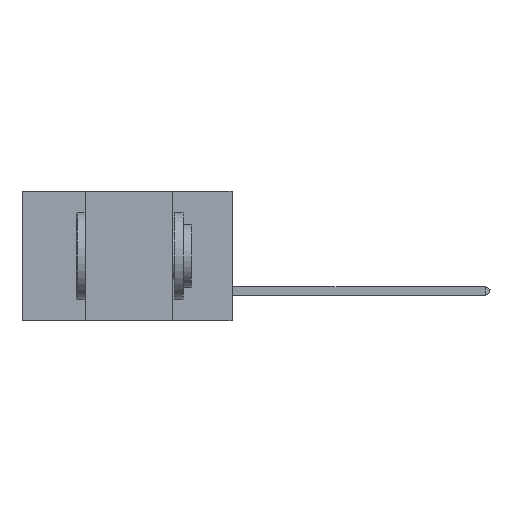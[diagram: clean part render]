
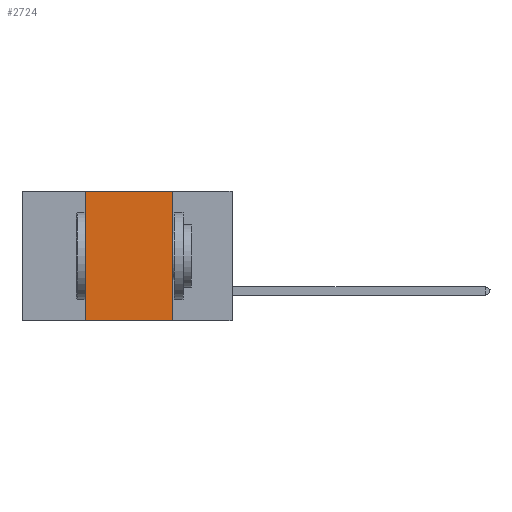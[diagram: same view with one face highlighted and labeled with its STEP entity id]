
A CAD part, left-side view. The second image highlights one B-rep face of the part: STEP entity #2724.
In plain terms, the highlighted planar face has unit normal (-1, 0, 0).
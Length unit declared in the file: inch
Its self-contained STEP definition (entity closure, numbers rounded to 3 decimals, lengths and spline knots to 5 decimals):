
#9 = CARTESIAN_POINT ( 'NONE',  ( 0., 0.42, 0. ) ) ;
#98 = LINE ( 'NONE', #13227, #13921 ) ;
#516 = EDGE_CURVE ( 'NONE', #10374, #6615, #3064, .T. ) ;
#602 = ORIENTED_EDGE ( 'NONE', *, *, #516, .F. ) ;
#1672 = VERTEX_POINT ( 'NONE', #12630 ) ;
#1884 = EDGE_CURVE ( 'NONE', #11666, #10374, #12898, .T. ) ;
#1972 = ORIENTED_EDGE ( 'NONE', *, *, #7058, .T. ) ;
#2417 = VECTOR ( 'NONE', #4203, 39.37008 ) ;
#2724 = ADVANCED_FACE ( 'NONE', ( #4492 ), #13463, .F. ) ;
#2881 = DIRECTION ( 'NONE',  ( 0., 0., -1. ) ) ;
#3064 = LINE ( 'NONE', #12149, #10852 ) ;
#3097 = CARTESIAN_POINT ( 'NONE',  ( 0., 0.42, 0. ) ) ;
#3380 = VECTOR ( 'NONE', #5176, 39.37008 ) ;
#4203 = DIRECTION ( 'NONE',  ( 0., 0., 1. ) ) ;
#4492 = FACE_OUTER_BOUND ( 'NONE', #13046, .T. ) ;
#5176 = DIRECTION ( 'NONE',  ( 0., -1., 0. ) ) ;
#5230 = CARTESIAN_POINT ( 'NONE',  ( 0., 0.6, 0. ) ) ;
#5797 = DIRECTION ( 'NONE',  ( 1., 0., 0. ) ) ;
#6615 = VERTEX_POINT ( 'NONE', #8226 ) ;
#7058 = EDGE_CURVE ( 'NONE', #1672, #6615, #98, .T. ) ;
#7242 = LINE ( 'NONE', #3097, #2417 ) ;
#7741 = DIRECTION ( 'NONE',  ( 0., -1., 0. ) ) ;
#8226 = CARTESIAN_POINT ( 'NONE',  ( 0., 0.17, -0.37 ) ) ;
#8994 = EDGE_CURVE ( 'NONE', #1672, #11666, #7242, .T. ) ;
#10236 = ORIENTED_EDGE ( 'NONE', *, *, #8994, .F. ) ;
#10374 = VERTEX_POINT ( 'NONE', #10829 ) ;
#10829 = CARTESIAN_POINT ( 'NONE',  ( 0., 0.17, 0. ) ) ;
#10852 = VECTOR ( 'NONE', #12203, 39.37008 ) ;
#11666 = VERTEX_POINT ( 'NONE', #9 ) ;
#12135 = ORIENTED_EDGE ( 'NONE', *, *, #1884, .F. ) ;
#12149 = CARTESIAN_POINT ( 'NONE',  ( 0., 0.17, 0. ) ) ;
#12203 = DIRECTION ( 'NONE',  ( 0., 0., -1. ) ) ;
#12630 = CARTESIAN_POINT ( 'NONE',  ( 0., 0.42, -0.37 ) ) ;
#12833 = AXIS2_PLACEMENT_3D ( 'NONE', #12865, #5797, #2881 ) ;
#12865 = CARTESIAN_POINT ( 'NONE',  ( 0., 0.6, 0. ) ) ;
#12898 = LINE ( 'NONE', #5230, #3380 ) ;
#13046 = EDGE_LOOP ( 'NONE', ( #602, #12135, #10236, #1972 ) ) ;
#13227 = CARTESIAN_POINT ( 'NONE',  ( 0., 0.6, -0.37 ) ) ;
#13463 = PLANE ( 'NONE',  #12833 ) ;
#13921 = VECTOR ( 'NONE', #7741, 39.37008 ) ;
